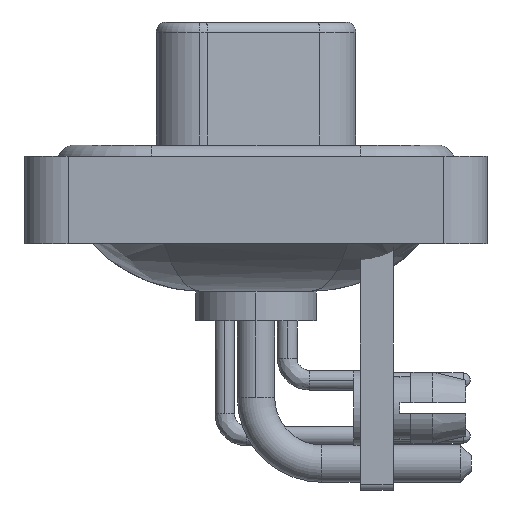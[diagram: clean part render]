
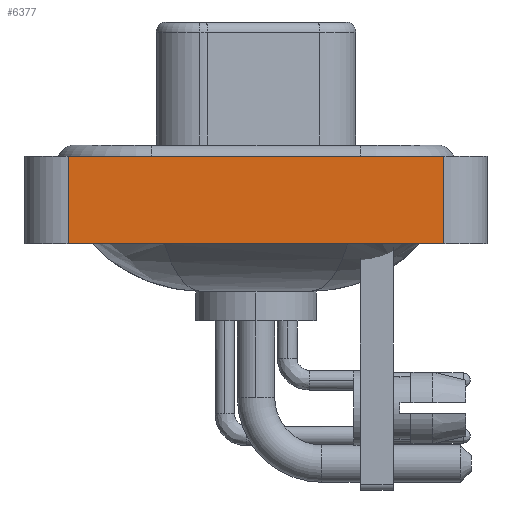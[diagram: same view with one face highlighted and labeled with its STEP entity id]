
A CAD part, left-side view. The second image highlights one B-rep face of the part: STEP entity #6377.
In plain terms, the highlighted planar face has unit normal (-1, 0, 0).
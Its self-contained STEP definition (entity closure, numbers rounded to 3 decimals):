
#706 = VECTOR ( 'NONE', #16818, 1000. ) ;
#1297 = DIRECTION ( 'NONE',  ( 0., 0., 1. ) ) ;
#1318 = EDGE_CURVE ( 'NONE', #21688, #24263, #26710, .T. ) ;
#2757 = CARTESIAN_POINT ( 'NONE',  ( -7.35, -8.55, -3.6 ) ) ;
#2904 = PLANE ( 'NONE',  #21233 ) ;
#4292 = CARTESIAN_POINT ( 'NONE',  ( -7.35, -8.55, -3.6 ) ) ;
#5080 = DIRECTION ( 'NONE',  ( -1., 0., 0. ) ) ;
#5243 = ORIENTED_EDGE ( 'NONE', *, *, #11614, .F. ) ;
#6377 = ADVANCED_FACE ( 'NONE', ( #24841 ), #2904, .T. ) ;
#7974 = CARTESIAN_POINT ( 'NONE',  ( -7.35, 8.55, -3.6 ) ) ;
#8127 = VECTOR ( 'NONE', #24405, 1000. ) ;
#9973 = DIRECTION ( 'NONE',  ( 0., 0., 1. ) ) ;
#10977 = CARTESIAN_POINT ( 'NONE',  ( -7.35, 8.55, -3.6 ) ) ;
#11253 = ORIENTED_EDGE ( 'NONE', *, *, #24218, .T. ) ;
#11425 = DIRECTION ( 'NONE',  ( 0., 0., 1. ) ) ;
#11614 = EDGE_CURVE ( 'NONE', #21688, #12335, #21368, .T. ) ;
#11835 = ORIENTED_EDGE ( 'NONE', *, *, #1318, .T. ) ;
#12335 = VERTEX_POINT ( 'NONE', #23168 ) ;
#12582 = CARTESIAN_POINT ( 'NONE',  ( -7.35, -8.55, 0.4 ) ) ;
#13401 = VECTOR ( 'NONE', #1297, 1000. ) ;
#14021 = VERTEX_POINT ( 'NONE', #12582 ) ;
#14128 = CARTESIAN_POINT ( 'NONE',  ( -7.35, -8.55, -3.6 ) ) ;
#14321 = EDGE_LOOP ( 'NONE', ( #11253, #14876, #5243, #11835 ) ) ;
#14876 = ORIENTED_EDGE ( 'NONE', *, *, #28420, .F. ) ;
#16818 = DIRECTION ( 'NONE',  ( 0., -1., 0. ) ) ;
#18813 = LINE ( 'NONE', #22879, #706 ) ;
#21233 = AXIS2_PLACEMENT_3D ( 'NONE', #22250, #5080, #11425 ) ;
#21368 = LINE ( 'NONE', #7974, #13401 ) ;
#21688 = VERTEX_POINT ( 'NONE', #10977 ) ;
#22250 = CARTESIAN_POINT ( 'NONE',  ( -7.35, -8.55, -3.6 ) ) ;
#22879 = CARTESIAN_POINT ( 'NONE',  ( -7.35, -8.55, 0.4 ) ) ;
#23073 = VECTOR ( 'NONE', #9973, 1000. ) ;
#23168 = CARTESIAN_POINT ( 'NONE',  ( -7.35, 8.55, 0.4 ) ) ;
#23375 = LINE ( 'NONE', #14128, #23073 ) ;
#24218 = EDGE_CURVE ( 'NONE', #24263, #14021, #23375, .T. ) ;
#24263 = VERTEX_POINT ( 'NONE', #4292 ) ;
#24405 = DIRECTION ( 'NONE',  ( 0., -1., 0. ) ) ;
#24841 = FACE_OUTER_BOUND ( 'NONE', #14321, .T. ) ;
#26710 = LINE ( 'NONE', #2757, #8127 ) ;
#28420 = EDGE_CURVE ( 'NONE', #12335, #14021, #18813, .T. ) ;
